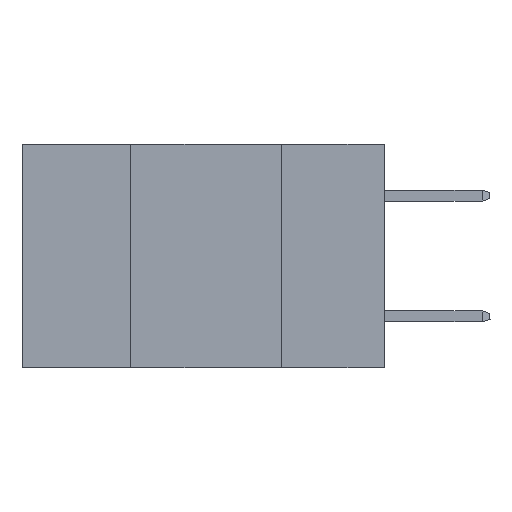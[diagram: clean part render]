
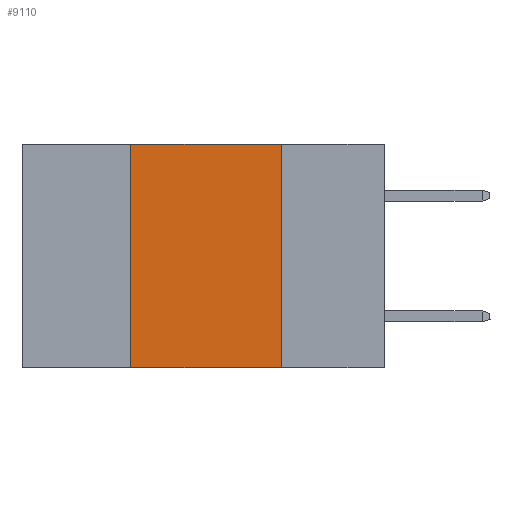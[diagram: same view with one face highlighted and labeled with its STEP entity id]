
A CAD part, left-side view. The second image highlights one B-rep face of the part: STEP entity #9110.
In plain terms, the highlighted planar face has unit normal (-1, 0, 0).
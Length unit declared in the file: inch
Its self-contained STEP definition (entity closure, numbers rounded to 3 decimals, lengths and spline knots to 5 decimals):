
#704 = DIRECTION ( 'NONE',  ( 0., 0., -1. ) ) ;
#971 = DIRECTION ( 'NONE',  ( 0., -1., 0. ) ) ;
#1207 = DIRECTION ( 'NONE',  ( 0., 0., 1. ) ) ;
#1759 = EDGE_CURVE ( 'NONE', #2969, #18792, #9753, .T. ) ;
#1795 = VECTOR ( 'NONE', #1207, 39.37008 ) ;
#2284 = EDGE_LOOP ( 'NONE', ( #4724, #17883, #13882, #9880 ) ) ;
#2969 = VERTEX_POINT ( 'NONE', #11211 ) ;
#3723 = PLANE ( 'NONE',  #12066 ) ;
#4303 = CARTESIAN_POINT ( 'NONE',  ( 0., 0.42, -0.37 ) ) ;
#4653 = CARTESIAN_POINT ( 'NONE',  ( 0., 0.17, -0.37 ) ) ;
#4724 = ORIENTED_EDGE ( 'NONE', *, *, #1759, .F. ) ;
#5252 = CARTESIAN_POINT ( 'NONE',  ( 0., 0.6, 0. ) ) ;
#5517 = DIRECTION ( 'NONE',  ( 0., 0., -1. ) ) ;
#5732 = CARTESIAN_POINT ( 'NONE',  ( 0., 0.17, -0.37 ) ) ;
#5799 = VECTOR ( 'NONE', #5517, 39.37008 ) ;
#7829 = VERTEX_POINT ( 'NONE', #14487 ) ;
#7984 = VERTEX_POINT ( 'NONE', #4303 ) ;
#9110 = ADVANCED_FACE ( 'NONE', ( #13929 ), #3723, .F. ) ;
#9753 = LINE ( 'NONE', #4653, #5799 ) ;
#9763 = DIRECTION ( 'NONE',  ( 1., 0., 0. ) ) ;
#9880 = ORIENTED_EDGE ( 'NONE', *, *, #16561, .T. ) ;
#10030 = CARTESIAN_POINT ( 'NONE',  ( 0., 0.6, -0.37 ) ) ;
#11211 = CARTESIAN_POINT ( 'NONE',  ( 0., 0.17, 0. ) ) ;
#11416 = LINE ( 'NONE', #15197, #14476 ) ;
#12066 = AXIS2_PLACEMENT_3D ( 'NONE', #5252, #9763, #704 ) ;
#12844 = EDGE_CURVE ( 'NONE', #7829, #2969, #11416, .T. ) ;
#13190 = VECTOR ( 'NONE', #971, 39.37008 ) ;
#13650 = LINE ( 'NONE', #10030, #13190 ) ;
#13882 = ORIENTED_EDGE ( 'NONE', *, *, #18061, .F. ) ;
#13929 = FACE_OUTER_BOUND ( 'NONE', #2284, .T. ) ;
#14476 = VECTOR ( 'NONE', #16729, 39.37008 ) ;
#14487 = CARTESIAN_POINT ( 'NONE',  ( 0., 0.42, 0. ) ) ;
#15197 = CARTESIAN_POINT ( 'NONE',  ( 0., 0.6, 0. ) ) ;
#16561 = EDGE_CURVE ( 'NONE', #7984, #18792, #13650, .T. ) ;
#16729 = DIRECTION ( 'NONE',  ( 0., -1., 0. ) ) ;
#17883 = ORIENTED_EDGE ( 'NONE', *, *, #12844, .F. ) ;
#18061 = EDGE_CURVE ( 'NONE', #7984, #7829, #18320, .T. ) ;
#18320 = LINE ( 'NONE', #19270, #1795 ) ;
#18792 = VERTEX_POINT ( 'NONE', #5732 ) ;
#19270 = CARTESIAN_POINT ( 'NONE',  ( 0., 0.42, -0.37 ) ) ;
